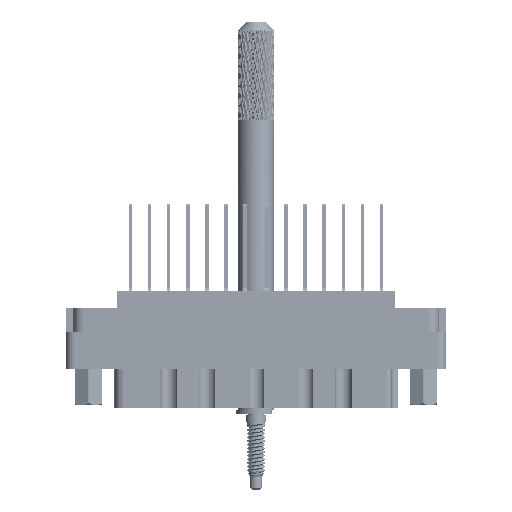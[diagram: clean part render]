
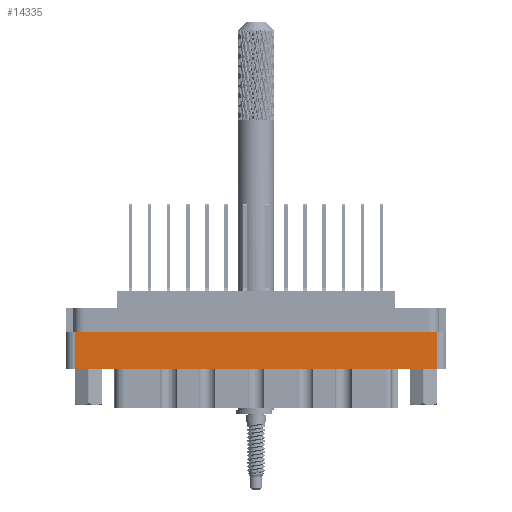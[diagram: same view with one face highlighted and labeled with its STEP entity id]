
A CAD part, front view. The second image highlights one B-rep face of the part: STEP entity #14335.
In plain terms, the highlighted planar face has unit normal (0, -1, 0).
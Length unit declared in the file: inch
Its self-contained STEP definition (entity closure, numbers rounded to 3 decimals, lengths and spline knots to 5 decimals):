
#6044 = VERTEX_POINT ( 'NONE', #73109 ) ;
#9023 = LINE ( 'NONE', #69932, #101651 ) ;
#10189 = FACE_OUTER_BOUND ( 'NONE', #21369, .T. ) ;
#12288 = ORIENTED_EDGE ( 'NONE', *, *, #103712, .T. ) ;
#12431 = ORIENTED_EDGE ( 'NONE', *, *, #16469, .F. ) ;
#14335 = ADVANCED_FACE ( 'NONE', ( #10189 ), #94072, .T. ) ;
#16469 = EDGE_CURVE ( 'NONE', #6044, #53771, #65948, .T. ) ;
#16480 = DIRECTION ( 'NONE',  ( 0., -1., 0. ) ) ;
#19732 = DIRECTION ( 'NONE',  ( 1., 0., 0. ) ) ;
#21369 = EDGE_LOOP ( 'NONE', ( #12431, #97645, #115078, #12288 ) ) ;
#21658 = DIRECTION ( 'NONE',  ( 0., 0., -1. ) ) ;
#23260 = CARTESIAN_POINT ( 'NONE',  ( 1.234, -0.438, -0.529 ) ) ;
#25834 = CARTESIAN_POINT ( 'NONE',  ( -1.296, -0.438, -0.798 ) ) ;
#35923 = EDGE_CURVE ( 'NONE', #89952, #78007, #45487, .T. ) ;
#40949 = VECTOR ( 'NONE', #121738, 39.37008 ) ;
#41279 = AXIS2_PLACEMENT_3D ( 'NONE', #25834, #16480, #66037 ) ;
#42925 = CARTESIAN_POINT ( 'NONE',  ( 0., -0.438, -0.529 ) ) ;
#45487 = LINE ( 'NONE', #42925, #40949 ) ;
#48957 = LINE ( 'NONE', #73721, #112750 ) ;
#53771 = VERTEX_POINT ( 'NONE', #82588 ) ;
#59837 = VECTOR ( 'NONE', #19732, 39.37008 ) ;
#62067 = CARTESIAN_POINT ( 'NONE',  ( -1.234, -0.438, -0.529 ) ) ;
#65103 = EDGE_CURVE ( 'NONE', #6044, #78007, #9023, .T. ) ;
#65948 = LINE ( 'NONE', #105366, #59837 ) ;
#66037 = DIRECTION ( 'NONE',  ( 0., 0., -1. ) ) ;
#69932 = CARTESIAN_POINT ( 'NONE',  ( -1.234, -0.438, -0.798 ) ) ;
#73109 = CARTESIAN_POINT ( 'NONE',  ( -1.234, -0.438, -0.277 ) ) ;
#73721 = CARTESIAN_POINT ( 'NONE',  ( 1.234, -0.438, -0.798 ) ) ;
#78007 = VERTEX_POINT ( 'NONE', #62067 ) ;
#82588 = CARTESIAN_POINT ( 'NONE',  ( 1.234, -0.438, -0.277 ) ) ;
#85556 = DIRECTION ( 'NONE',  ( 0., 0., 1. ) ) ;
#89952 = VERTEX_POINT ( 'NONE', #23260 ) ;
#94072 = PLANE ( 'NONE',  #41279 ) ;
#97645 = ORIENTED_EDGE ( 'NONE', *, *, #65103, .T. ) ;
#101651 = VECTOR ( 'NONE', #21658, 39.37008 ) ;
#103712 = EDGE_CURVE ( 'NONE', #89952, #53771, #48957, .T. ) ;
#105366 = CARTESIAN_POINT ( 'NONE',  ( 0., -0.438, -0.277 ) ) ;
#112750 = VECTOR ( 'NONE', #85556, 39.37008 ) ;
#115078 = ORIENTED_EDGE ( 'NONE', *, *, #35923, .F. ) ;
#121738 = DIRECTION ( 'NONE',  ( -1., 0., 0. ) ) ;
